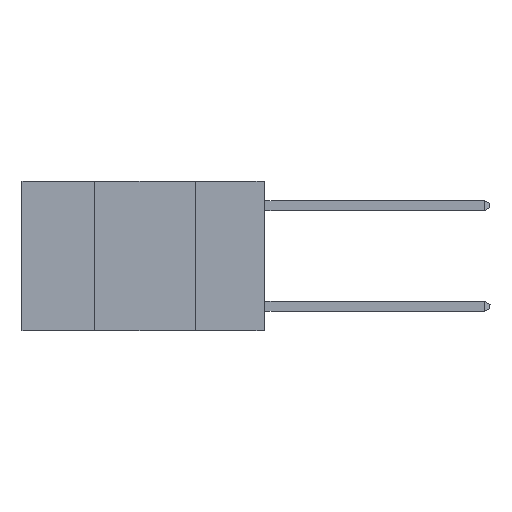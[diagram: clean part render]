
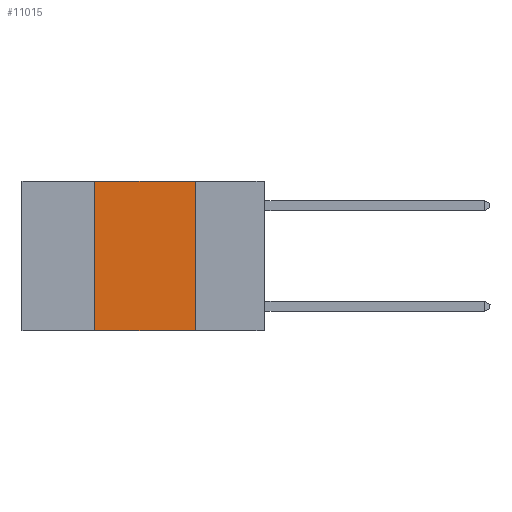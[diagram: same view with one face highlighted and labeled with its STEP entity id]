
A CAD part, left-side view. The second image highlights one B-rep face of the part: STEP entity #11015.
In plain terms, the highlighted planar face has unit normal (-1, 0, 0).
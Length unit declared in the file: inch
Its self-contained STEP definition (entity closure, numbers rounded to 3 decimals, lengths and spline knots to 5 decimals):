
#134 = CARTESIAN_POINT ( 'NONE',  ( 0., 0.42, 0. ) ) ;
#403 = CARTESIAN_POINT ( 'NONE',  ( 0., 0.6, -0.37 ) ) ;
#1290 = DIRECTION ( 'NONE',  ( 0., -1., 0. ) ) ;
#1824 = PLANE ( 'NONE',  #27021 ) ;
#2956 = DIRECTION ( 'NONE',  ( 0., -1., 0. ) ) ;
#3569 = CARTESIAN_POINT ( 'NONE',  ( 0., 0.42, -0.37 ) ) ;
#3688 = EDGE_CURVE ( 'NONE', #21363, #5834, #20048, .T. ) ;
#4387 = CARTESIAN_POINT ( 'NONE',  ( 0., 0.6, 0. ) ) ;
#5834 = VERTEX_POINT ( 'NONE', #13743 ) ;
#6788 = VECTOR ( 'NONE', #2956, 39.37008 ) ;
#6913 = DIRECTION ( 'NONE',  ( 1., 0., 0. ) ) ;
#7315 = CARTESIAN_POINT ( 'NONE',  ( 0., 0.17, 0. ) ) ;
#7578 = LINE ( 'NONE', #403, #6788 ) ;
#8185 = CARTESIAN_POINT ( 'NONE',  ( 0., 0.42, 0. ) ) ;
#8917 = EDGE_CURVE ( 'NONE', #21608, #21363, #26652, .T. ) ;
#10549 = ORIENTED_EDGE ( 'NONE', *, *, #3688, .F. ) ;
#11015 = ADVANCED_FACE ( 'NONE', ( #29971 ), #1824, .F. ) ;
#12114 = ORIENTED_EDGE ( 'NONE', *, *, #15136, .F. ) ;
#12689 = EDGE_LOOP ( 'NONE', ( #10549, #23840, #12114, #31977 ) ) ;
#13451 = VERTEX_POINT ( 'NONE', #3569 ) ;
#13743 = CARTESIAN_POINT ( 'NONE',  ( 0., 0.17, -0.37 ) ) ;
#15136 = EDGE_CURVE ( 'NONE', #13451, #21608, #25807, .T. ) ;
#15205 = CARTESIAN_POINT ( 'NONE',  ( 0., 0.17, 0. ) ) ;
#15221 = DIRECTION ( 'NONE',  ( 0., 0., 1. ) ) ;
#18470 = VECTOR ( 'NONE', #30142, 39.37008 ) ;
#19169 = VECTOR ( 'NONE', #15221, 39.37008 ) ;
#19994 = VECTOR ( 'NONE', #1290, 39.37008 ) ;
#20048 = LINE ( 'NONE', #15205, #18470 ) ;
#21363 = VERTEX_POINT ( 'NONE', #7315 ) ;
#21608 = VERTEX_POINT ( 'NONE', #8185 ) ;
#22271 = EDGE_CURVE ( 'NONE', #13451, #5834, #7578, .T. ) ;
#23777 = CARTESIAN_POINT ( 'NONE',  ( 0., 0.6, 0. ) ) ;
#23840 = ORIENTED_EDGE ( 'NONE', *, *, #8917, .F. ) ;
#24427 = DIRECTION ( 'NONE',  ( 0., 0., -1. ) ) ;
#25807 = LINE ( 'NONE', #134, #19169 ) ;
#26652 = LINE ( 'NONE', #23777, #19994 ) ;
#27021 = AXIS2_PLACEMENT_3D ( 'NONE', #4387, #6913, #24427 ) ;
#29971 = FACE_OUTER_BOUND ( 'NONE', #12689, .T. ) ;
#30142 = DIRECTION ( 'NONE',  ( 0., 0., -1. ) ) ;
#31977 = ORIENTED_EDGE ( 'NONE', *, *, #22271, .T. ) ;
